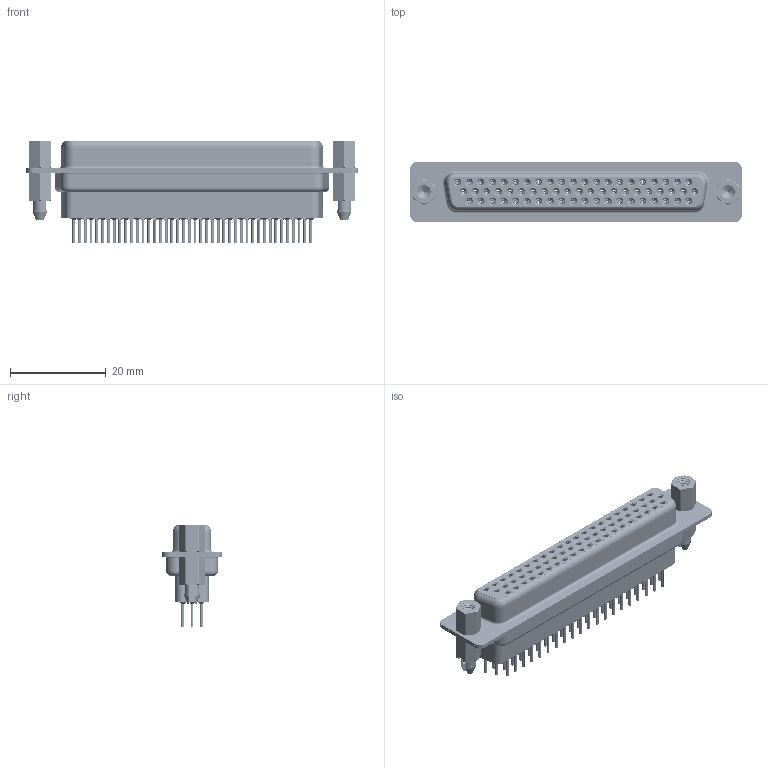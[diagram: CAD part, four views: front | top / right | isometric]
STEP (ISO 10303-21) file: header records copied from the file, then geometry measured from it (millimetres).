
FILE_DESCRIPTION (( 'STEP AP203' ), '1' );
FILE_NAME ('638-062-331-077.STEP', '2020-07-19T01:58:51', ( '' ), ( '' ), 'SwSTEP 2.0', 'SolidWorks 2020', '' );
FILE_SCHEMA (( 'CONFIG_CONTROL_DESIGN' ));
Length unit declared in the file: millimetre
Products named in the file (9): 638 Contact Row 3_31; 638 4-40 Threaded Boardlock_LP; 638-062-331-077; 638 Shell Front_62 Contacts; 638 Contact Row 2_31; 638 4-40 Hex Standoff; 638 Shell Rear_62 Contacts; 638 Contact Row 1_31; 638 Housing_62 Contacts HP
Assembly tree (69 placements, depth 2):
  638-062-331-077
    638 Housing_62 Contacts HP
    638 Shell Front_62 Contacts
    638 Shell Rear_62 Contacts
    638 Contact Row 1_31  x21
    638 Contact Row 2_31  x21
    638 Contact Row 3_31  x20
    638 4-40 Hex Standoff  x2
    638 4-40 Threaded Boardlock_LP  x2
Bounding box: 69.32 x 12.6 x 21.5 mm (x, y, z)
Volume: 5967.7 mm3; surface area: 21886 mm2
Topology: 69 solids, 69 shells, 8105 faces, 20857 edges, 13023 vertices
Faces by surface type: cylinder 2287, plane 2043, torus 1545, bspline 1258, cone 972
Entity records: 52710 total; most frequent: CARTESIAN_POINT 15259, DIRECTION 7716, ORIENTED_EDGE 6978, EDGE_CURVE 3489, AXIS2_PLACEMENT_3D 3244, VERTEX_POINT 2219, EDGE_LOOP 1816, CIRCLE 1759
